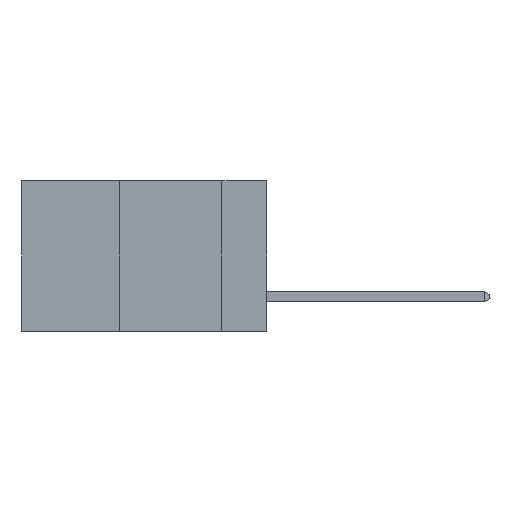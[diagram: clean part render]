
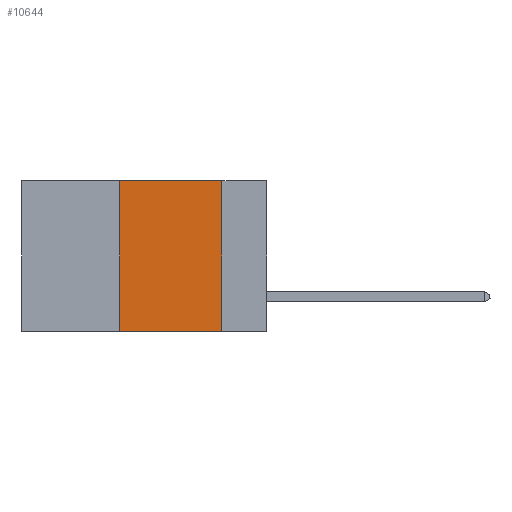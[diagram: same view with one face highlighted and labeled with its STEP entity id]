
A CAD part, left-side view. The second image highlights one B-rep face of the part: STEP entity #10644.
In plain terms, the highlighted planar face has unit normal (-1, 0, 0).
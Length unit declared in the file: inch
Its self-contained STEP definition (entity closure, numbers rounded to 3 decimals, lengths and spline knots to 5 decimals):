
#589 = CARTESIAN_POINT ( 'NONE',  ( 0., 0.36, 0. ) ) ;
#1221 = VERTEX_POINT ( 'NONE', #15279 ) ;
#1908 = VECTOR ( 'NONE', #21232, 39.37008 ) ;
#2837 = PLANE ( 'NONE',  #10577 ) ;
#3557 = LINE ( 'NONE', #8411, #1908 ) ;
#4876 = VERTEX_POINT ( 'NONE', #19902 ) ;
#6243 = DIRECTION ( 'NONE',  ( 0., 0., -1. ) ) ;
#8411 = CARTESIAN_POINT ( 'NONE',  ( 0., 0.6, -0.37 ) ) ;
#10298 = VERTEX_POINT ( 'NONE', #13580 ) ;
#10577 = AXIS2_PLACEMENT_3D ( 'NONE', #20149, #18233, #6243 ) ;
#10644 = ADVANCED_FACE ( 'NONE', ( #21089 ), #2837, .F. ) ;
#11176 = DIRECTION ( 'NONE',  ( 0., 0., -1. ) ) ;
#12836 = EDGE_CURVE ( 'NONE', #10298, #1221, #17444, .T. ) ;
#12846 = ORIENTED_EDGE ( 'NONE', *, *, #14349, .T. ) ;
#13580 = CARTESIAN_POINT ( 'NONE',  ( 0., 0.11, 0. ) ) ;
#13929 = EDGE_LOOP ( 'NONE', ( #18630, #20251, #19233, #12846 ) ) ;
#14349 = EDGE_CURVE ( 'NONE', #15150, #1221, #3557, .T. ) ;
#15150 = VERTEX_POINT ( 'NONE', #16124 ) ;
#15279 = CARTESIAN_POINT ( 'NONE',  ( 0., 0.11, -0.37 ) ) ;
#15881 = EDGE_CURVE ( 'NONE', #4876, #10298, #16669, .T. ) ;
#15969 = DIRECTION ( 'NONE',  ( 0., -1., 0. ) ) ;
#16124 = CARTESIAN_POINT ( 'NONE',  ( 0., 0.36, -0.37 ) ) ;
#16185 = LINE ( 'NONE', #589, #19172 ) ;
#16669 = LINE ( 'NONE', #17559, #19687 ) ;
#17444 = LINE ( 'NONE', #19930, #21240 ) ;
#17559 = CARTESIAN_POINT ( 'NONE',  ( 0., 0.6, 0. ) ) ;
#17979 = DIRECTION ( 'NONE',  ( 0., 0., 1. ) ) ;
#18233 = DIRECTION ( 'NONE',  ( 1., 0., 0. ) ) ;
#18630 = ORIENTED_EDGE ( 'NONE', *, *, #12836, .F. ) ;
#19172 = VECTOR ( 'NONE', #17979, 39.37008 ) ;
#19233 = ORIENTED_EDGE ( 'NONE', *, *, #21309, .F. ) ;
#19687 = VECTOR ( 'NONE', #15969, 39.37008 ) ;
#19902 = CARTESIAN_POINT ( 'NONE',  ( 0., 0.36, 0. ) ) ;
#19930 = CARTESIAN_POINT ( 'NONE',  ( 0., 0.11, 0. ) ) ;
#20149 = CARTESIAN_POINT ( 'NONE',  ( 0., 0.6, 0. ) ) ;
#20251 = ORIENTED_EDGE ( 'NONE', *, *, #15881, .F. ) ;
#21089 = FACE_OUTER_BOUND ( 'NONE', #13929, .T. ) ;
#21232 = DIRECTION ( 'NONE',  ( 0., -1., 0. ) ) ;
#21240 = VECTOR ( 'NONE', #11176, 39.37008 ) ;
#21309 = EDGE_CURVE ( 'NONE', #15150, #4876, #16185, .T. ) ;
